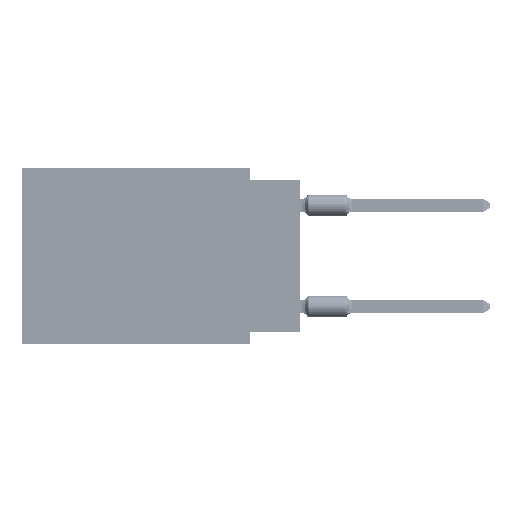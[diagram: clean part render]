
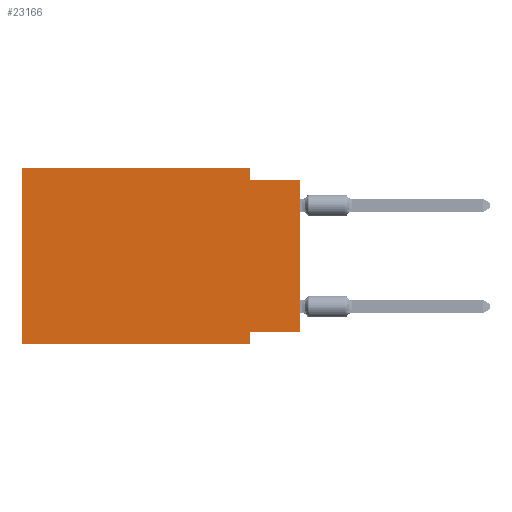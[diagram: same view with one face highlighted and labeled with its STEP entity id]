
A CAD part, left-side view. The second image highlights one B-rep face of the part: STEP entity #23166.
In plain terms, the highlighted planar face has unit normal (-1, 0, 0).
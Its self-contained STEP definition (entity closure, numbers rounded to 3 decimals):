
#1641 = DIRECTION ( 'NONE',  ( 0., 0., 1. ) ) ;
#2768 = VECTOR ( 'NONE', #74813, 1000. ) ;
#3011 = ORIENTED_EDGE ( 'NONE', *, *, #69035, .F. ) ;
#3351 = CARTESIAN_POINT ( 'NONE',  ( 0., 13.97, 0. ) ) ;
#3667 = ORIENTED_EDGE ( 'NONE', *, *, #72526, .F. ) ;
#5470 = ORIENTED_EDGE ( 'NONE', *, *, #62305, .T. ) ;
#6791 = CARTESIAN_POINT ( 'NONE',  ( 0., 0., -8.255 ) ) ;
#7620 = ORIENTED_EDGE ( 'NONE', *, *, #52630, .F. ) ;
#7822 = LINE ( 'NONE', #21002, #63218 ) ;
#8110 = LINE ( 'NONE', #69566, #47270 ) ;
#8595 = VERTEX_POINT ( 'NONE', #47139 ) ;
#12167 = DIRECTION ( 'NONE',  ( 0., 1., 0. ) ) ;
#12666 = DIRECTION ( 'NONE',  ( 0., 0., -1. ) ) ;
#12845 = CARTESIAN_POINT ( 'NONE',  ( 0., 2.54, -0.635 ) ) ;
#13383 = DIRECTION ( 'NONE',  ( 0., -1., 0. ) ) ;
#15004 = DIRECTION ( 'NONE',  ( 0., 0., -1. ) ) ;
#16601 = EDGE_CURVE ( 'NONE', #61826, #77609, #44747, .T. ) ;
#18816 = CARTESIAN_POINT ( 'NONE',  ( 0., 13.97, 0. ) ) ;
#20907 = EDGE_CURVE ( 'NONE', #32885, #29557, #23142, .T. ) ;
#21002 = CARTESIAN_POINT ( 'NONE',  ( 0., 13.97, 0. ) ) ;
#23142 = LINE ( 'NONE', #3351, #55383 ) ;
#23166 = ADVANCED_FACE ( 'NONE', ( #36979 ), #25805, .F. ) ;
#25805 = PLANE ( 'NONE',  #27927 ) ;
#26159 = VERTEX_POINT ( 'NONE', #12845 ) ;
#27927 = AXIS2_PLACEMENT_3D ( 'NONE', #18816, #63345, #42749 ) ;
#29557 = VERTEX_POINT ( 'NONE', #52366 ) ;
#32885 = VERTEX_POINT ( 'NONE', #77814 ) ;
#33444 = LINE ( 'NONE', #65584, #75301 ) ;
#33976 = CARTESIAN_POINT ( 'NONE',  ( 0., 2.54, -8.89 ) ) ;
#36979 = FACE_OUTER_BOUND ( 'NONE', #48480, .T. ) ;
#40542 = CARTESIAN_POINT ( 'NONE',  ( 0., 2.54, -8.255 ) ) ;
#40816 = EDGE_CURVE ( 'NONE', #78690, #32885, #7822, .T. ) ;
#42272 = LINE ( 'NONE', #80583, #2768 ) ;
#42749 = DIRECTION ( 'NONE',  ( 0., 0., -1. ) ) ;
#43867 = ORIENTED_EDGE ( 'NONE', *, *, #20907, .F. ) ;
#44747 = LINE ( 'NONE', #6791, #57748 ) ;
#44751 = LINE ( 'NONE', #69871, #72041 ) ;
#45570 = LINE ( 'NONE', #33976, #74437 ) ;
#45661 = CARTESIAN_POINT ( 'NONE',  ( 0., 0., -8.255 ) ) ;
#47139 = CARTESIAN_POINT ( 'NONE',  ( 0., 0., -0.635 ) ) ;
#47270 = VECTOR ( 'NONE', #12666, 1000. ) ;
#47878 = ORIENTED_EDGE ( 'NONE', *, *, #16601, .F. ) ;
#48480 = EDGE_LOOP ( 'NONE', ( #59503, #3011, #7620, #43867, #73413, #5470, #3667, #47878 ) ) ;
#52366 = CARTESIAN_POINT ( 'NONE',  ( 0., 2.54, 0. ) ) ;
#52630 = EDGE_CURVE ( 'NONE', #29557, #26159, #8110, .T. ) ;
#55383 = VECTOR ( 'NONE', #72629, 1000. ) ;
#57748 = VECTOR ( 'NONE', #12167, 1000. ) ;
#59503 = ORIENTED_EDGE ( 'NONE', *, *, #69722, .T. ) ;
#61826 = VERTEX_POINT ( 'NONE', #45661 ) ;
#62305 = EDGE_CURVE ( 'NONE', #78690, #63547, #44751, .T. ) ;
#63218 = VECTOR ( 'NONE', #1641, 1000. ) ;
#63345 = DIRECTION ( 'NONE',  ( 1., 0., 0. ) ) ;
#63547 = VERTEX_POINT ( 'NONE', #72724 ) ;
#65584 = CARTESIAN_POINT ( 'NONE',  ( 0., 0., 0. ) ) ;
#69035 = EDGE_CURVE ( 'NONE', #26159, #8595, #42272, .T. ) ;
#69566 = CARTESIAN_POINT ( 'NONE',  ( 0., 2.54, 0. ) ) ;
#69722 = EDGE_CURVE ( 'NONE', #61826, #8595, #33444, .T. ) ;
#69871 = CARTESIAN_POINT ( 'NONE',  ( 0., 13.97, -8.89 ) ) ;
#72041 = VECTOR ( 'NONE', #13383, 1000. ) ;
#72526 = EDGE_CURVE ( 'NONE', #77609, #63547, #45570, .T. ) ;
#72629 = DIRECTION ( 'NONE',  ( 0., -1., 0. ) ) ;
#72724 = CARTESIAN_POINT ( 'NONE',  ( 0., 2.54, -8.89 ) ) ;
#73413 = ORIENTED_EDGE ( 'NONE', *, *, #40816, .F. ) ;
#73647 = CARTESIAN_POINT ( 'NONE',  ( 0., 13.97, -8.89 ) ) ;
#74437 = VECTOR ( 'NONE', #15004, 1000. ) ;
#74813 = DIRECTION ( 'NONE',  ( 0., -1., 0. ) ) ;
#75301 = VECTOR ( 'NONE', #77541, 1000. ) ;
#77541 = DIRECTION ( 'NONE',  ( 0., 0., 1. ) ) ;
#77609 = VERTEX_POINT ( 'NONE', #40542 ) ;
#77814 = CARTESIAN_POINT ( 'NONE',  ( 0., 13.97, 0. ) ) ;
#78690 = VERTEX_POINT ( 'NONE', #73647 ) ;
#80583 = CARTESIAN_POINT ( 'NONE',  ( 0., 0., -0.635 ) ) ;
